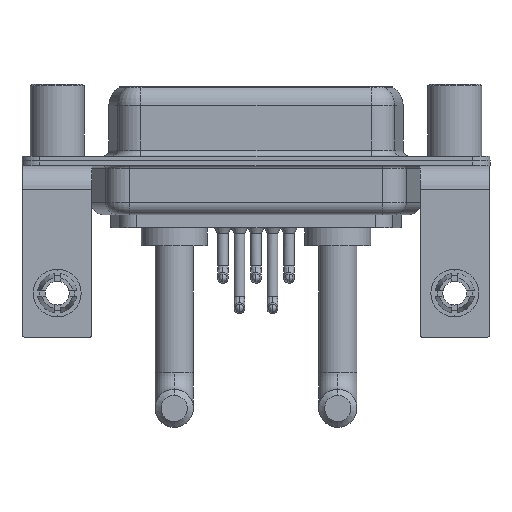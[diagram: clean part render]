
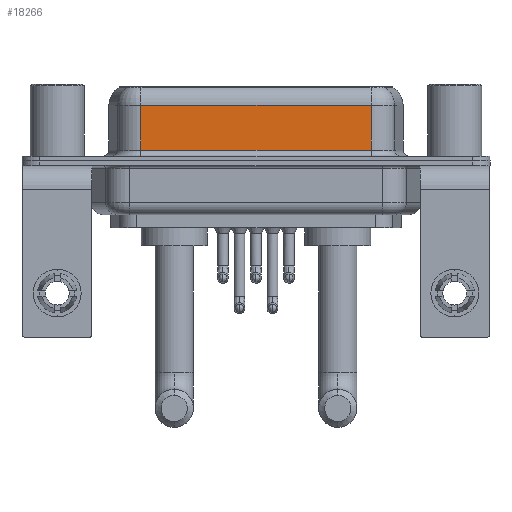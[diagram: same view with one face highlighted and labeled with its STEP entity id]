
A CAD part, front view. The second image highlights one B-rep face of the part: STEP entity #18266.
In plain terms, the highlighted planar face has unit normal (0, -1, 0).
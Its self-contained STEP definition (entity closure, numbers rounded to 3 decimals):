
#264 = ORIENTED_EDGE ( 'NONE', *, *, #11228, .T. ) ;
#1237 = DIRECTION ( 'NONE',  ( 1., 0., 0. ) ) ;
#1355 = VECTOR ( 'NONE', #4785, 1000. ) ;
#1777 = CARTESIAN_POINT ( 'NONE',  ( 7.013, -3.95, 0.9 ) ) ;
#1789 = ORIENTED_EDGE ( 'NONE', *, *, #2965, .F. ) ;
#1959 = CARTESIAN_POINT ( 'NONE',  ( 26.287, -3.95, 6.4 ) ) ;
#2418 = ORIENTED_EDGE ( 'NONE', *, *, #14768, .T. ) ;
#2965 = EDGE_CURVE ( 'NONE', #10047, #8305, #8010, .T. ) ;
#3569 = DIRECTION ( 'NONE',  ( 0., 1., 0. ) ) ;
#4785 = DIRECTION ( 'NONE',  ( -1., 0., 0. ) ) ;
#5459 = LINE ( 'NONE', #11942, #11461 ) ;
#6358 = EDGE_CURVE ( 'NONE', #13927, #8305, #12186, .T. ) ;
#6487 = CARTESIAN_POINT ( 'NONE',  ( 7.013, -3.95, 4.65 ) ) ;
#6942 = DIRECTION ( 'NONE',  ( 0., 0., -1. ) ) ;
#7291 = CARTESIAN_POINT ( 'NONE',  ( 26.287, -3.95, 0.9 ) ) ;
#8010 = LINE ( 'NONE', #1959, #16369 ) ;
#8305 = VERTEX_POINT ( 'NONE', #17365 ) ;
#8916 = AXIS2_PLACEMENT_3D ( 'NONE', #18133, #3569, #16539 ) ;
#9514 = EDGE_LOOP ( 'NONE', ( #1789, #2418, #264, #13487 ) ) ;
#9562 = LINE ( 'NONE', #15951, #1355 ) ;
#10047 = VERTEX_POINT ( 'NONE', #10535 ) ;
#10535 = CARTESIAN_POINT ( 'NONE',  ( 26.287, -3.95, 4.65 ) ) ;
#11228 = EDGE_CURVE ( 'NONE', #14897, #13927, #5459, .T. ) ;
#11461 = VECTOR ( 'NONE', #6942, 1000. ) ;
#11942 = CARTESIAN_POINT ( 'NONE',  ( 7.013, -3.95, 6.4 ) ) ;
#12186 = LINE ( 'NONE', #7291, #19560 ) ;
#13436 = DIRECTION ( 'NONE',  ( 0., 0., -1. ) ) ;
#13487 = ORIENTED_EDGE ( 'NONE', *, *, #6358, .T. ) ;
#13927 = VERTEX_POINT ( 'NONE', #1777 ) ;
#14725 = FACE_OUTER_BOUND ( 'NONE', #9514, .T. ) ;
#14768 = EDGE_CURVE ( 'NONE', #10047, #14897, #9562, .T. ) ;
#14826 = PLANE ( 'NONE',  #8916 ) ;
#14897 = VERTEX_POINT ( 'NONE', #6487 ) ;
#15951 = CARTESIAN_POINT ( 'NONE',  ( 26.287, -3.95, 4.65 ) ) ;
#16369 = VECTOR ( 'NONE', #13436, 1000. ) ;
#16539 = DIRECTION ( 'NONE',  ( 0., 0., 1. ) ) ;
#17365 = CARTESIAN_POINT ( 'NONE',  ( 26.287, -3.95, 0.9 ) ) ;
#18133 = CARTESIAN_POINT ( 'NONE',  ( 26.287, -3.95, 6.4 ) ) ;
#18266 = ADVANCED_FACE ( 'NONE', ( #14725 ), #14826, .F. ) ;
#19560 = VECTOR ( 'NONE', #1237, 1000. ) ;
